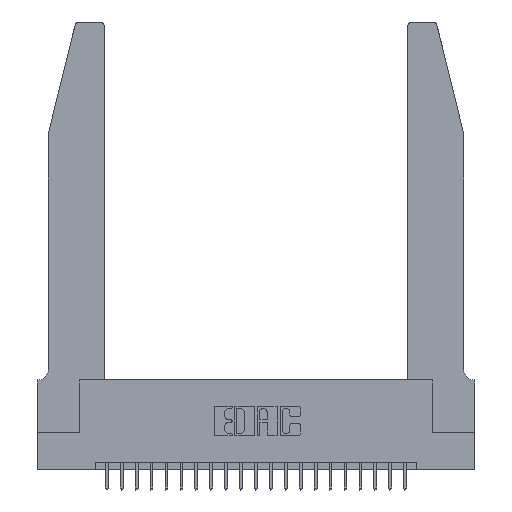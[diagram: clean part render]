
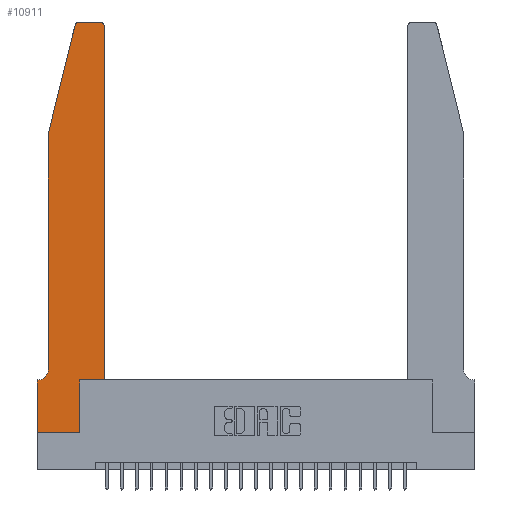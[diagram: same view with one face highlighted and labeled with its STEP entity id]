
A CAD part, top view. The second image highlights one B-rep face of the part: STEP entity #10911.
In plain terms, the highlighted planar face has unit normal (0, 0, 1).
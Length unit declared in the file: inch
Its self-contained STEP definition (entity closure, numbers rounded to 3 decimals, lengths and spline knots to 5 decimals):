
#308 = VERTEX_POINT ( 'NONE', #14367 ) ;
#468 = CARTESIAN_POINT ( 'NONE',  ( 0.2865, 0., 0.37 ) ) ;
#520 = VERTEX_POINT ( 'NONE', #7309 ) ;
#607 = FACE_OUTER_BOUND ( 'NONE', #18748, .T. ) ;
#777 = CARTESIAN_POINT ( 'NONE',  ( 0.0755, 2., 0.37 ) ) ;
#827 = ORIENTED_EDGE ( 'NONE', *, *, #13440, .T. ) ;
#828 = ORIENTED_EDGE ( 'NONE', *, *, #21350, .T. ) ;
#1389 = CARTESIAN_POINT ( 'NONE',  ( 0., 0.35, 0.37 ) ) ;
#1522 = ORIENTED_EDGE ( 'NONE', *, *, #9879, .T. ) ;
#1640 = LINE ( 'NONE', #20611, #9309 ) ;
#1994 = CIRCLE ( 'NONE', #5898, 0.03 ) ;
#2010 = CARTESIAN_POINT ( 'NONE',  ( 0.2605, 2.75, 0.37 ) ) ;
#2031 = CARTESIAN_POINT ( 'NONE',  ( 0., 0., 0.37 ) ) ;
#2139 = ORIENTED_EDGE ( 'NONE', *, *, #13582, .T. ) ;
#2393 = DIRECTION ( 'NONE',  ( 0., 0., -1. ) ) ;
#2446 = ORIENTED_EDGE ( 'NONE', *, *, #19877, .T. ) ;
#3504 = VECTOR ( 'NONE', #11298, 39.37008 ) ;
#3564 = EDGE_CURVE ( 'NONE', #520, #5819, #19365, .T. ) ;
#4402 = PLANE ( 'NONE',  #9981 ) ;
#4574 = VERTEX_POINT ( 'NONE', #468 ) ;
#5304 = ORIENTED_EDGE ( 'NONE', *, *, #3564, .T. ) ;
#5811 = ORIENTED_EDGE ( 'NONE', *, *, #16252, .T. ) ;
#5819 = VERTEX_POINT ( 'NONE', #8015 ) ;
#5851 = CIRCLE ( 'NONE', #16009, 0.03 ) ;
#5898 = AXIS2_PLACEMENT_3D ( 'NONE', #21106, #11808, #18772 ) ;
#6084 = VECTOR ( 'NONE', #6490, 39.37008 ) ;
#6261 = CARTESIAN_POINT ( 'NONE',  ( 0.4505, 0.35, 0.37 ) ) ;
#6490 = DIRECTION ( 'NONE',  ( 0., -1., 0. ) ) ;
#7309 = CARTESIAN_POINT ( 'NONE',  ( 0.0755, 0.42, 0.37 ) ) ;
#7367 = DIRECTION ( 'NONE',  ( -0.239, -0.971, 0. ) ) ;
#7811 = EDGE_CURVE ( 'NONE', #308, #12737, #1640, .T. ) ;
#7961 = CARTESIAN_POINT ( 'NONE',  ( 0., 0.35, 0.37 ) ) ;
#8015 = CARTESIAN_POINT ( 'NONE',  ( 0.0055, 0.35, 0.37 ) ) ;
#8226 = DIRECTION ( 'NONE',  ( 0., 1., 0. ) ) ;
#8350 = VERTEX_POINT ( 'NONE', #10363 ) ;
#8658 = LINE ( 'NONE', #16139, #16761 ) ;
#8765 = DIRECTION ( 'NONE',  ( -1., 0., 0. ) ) ;
#8970 = ORIENTED_EDGE ( 'NONE', *, *, #22170, .T. ) ;
#9088 = VERTEX_POINT ( 'NONE', #13491 ) ;
#9309 = VECTOR ( 'NONE', #7367, 39.37008 ) ;
#9360 = ORIENTED_EDGE ( 'NONE', *, *, #16908, .T. ) ;
#9458 = DIRECTION ( 'NONE',  ( -1., 0., 0. ) ) ;
#9585 = LINE ( 'NONE', #6261, #21697 ) ;
#9609 = VECTOR ( 'NONE', #9458, 39.37008 ) ;
#9879 = EDGE_CURVE ( 'NONE', #8350, #10273, #9585, .T. ) ;
#9981 = AXIS2_PLACEMENT_3D ( 'NONE', #7961, #15685, #15196 ) ;
#10273 = VERTEX_POINT ( 'NONE', #16044 ) ;
#10363 = CARTESIAN_POINT ( 'NONE',  ( 0.4505, 0.35, 0.37 ) ) ;
#10710 = DIRECTION ( 'NONE',  ( 0., -1., 0. ) ) ;
#10911 = ADVANCED_FACE ( 'NONE', ( #607 ), #4402, .T. ) ;
#11044 = LINE ( 'NONE', #18856, #3504 ) ;
#11298 = DIRECTION ( 'NONE',  ( 0., 1., 0. ) ) ;
#11535 = CARTESIAN_POINT ( 'NONE',  ( 0.0755, 0.35, 0.37 ) ) ;
#11569 = AXIS2_PLACEMENT_3D ( 'NONE', #19142, #2393, #8765 ) ;
#11808 = DIRECTION ( 'NONE',  ( 0., 0., 1. ) ) ;
#12515 = VECTOR ( 'NONE', #17495, 39.37008 ) ;
#12737 = VERTEX_POINT ( 'NONE', #777 ) ;
#12916 = LINE ( 'NONE', #16358, #16746 ) ;
#13222 = LINE ( 'NONE', #17130, #20386 ) ;
#13440 = EDGE_CURVE ( 'NONE', #19111, #23696, #18757, .T. ) ;
#13491 = CARTESIAN_POINT ( 'NONE',  ( 0.2865, 0.35, 0.37 ) ) ;
#13582 = EDGE_CURVE ( 'NONE', #12737, #520, #23620, .T. ) ;
#14234 = ORIENTED_EDGE ( 'NONE', *, *, #17734, .T. ) ;
#14367 = CARTESIAN_POINT ( 'NONE',  ( 0.25487, 2.72718, 0.37 ) ) ;
#14754 = DIRECTION ( 'NONE',  ( 1., 0., 0. ) ) ;
#15132 = CARTESIAN_POINT ( 'NONE',  ( 0.4205, 2.75, 0.37 ) ) ;
#15196 = DIRECTION ( 'NONE',  ( 1., 0., 0. ) ) ;
#15685 = DIRECTION ( 'NONE',  ( 0., 0., 1. ) ) ;
#15788 = LINE ( 'NONE', #11535, #12515 ) ;
#16009 = AXIS2_PLACEMENT_3D ( 'NONE', #20029, #20148, #14754 ) ;
#16044 = CARTESIAN_POINT ( 'NONE',  ( 0.4505, 2.72, 0.37 ) ) ;
#16062 = ORIENTED_EDGE ( 'NONE', *, *, #7811, .T. ) ;
#16139 = CARTESIAN_POINT ( 'NONE',  ( 0., 0., 0.37 ) ) ;
#16184 = CARTESIAN_POINT ( 'NONE',  ( 0.0755, 2., 0.37 ) ) ;
#16252 = EDGE_CURVE ( 'NONE', #18072, #22385, #12916, .T. ) ;
#16358 = CARTESIAN_POINT ( 'NONE',  ( 0., 0., 0.37 ) ) ;
#16746 = VECTOR ( 'NONE', #10710, 39.37008 ) ;
#16761 = VECTOR ( 'NONE', #23573, 39.37008 ) ;
#16894 = DIRECTION ( 'NONE',  ( 1., 0., 0. ) ) ;
#16908 = EDGE_CURVE ( 'NONE', #22385, #4574, #8658, .T. ) ;
#17130 = CARTESIAN_POINT ( 'NONE',  ( 0.4505, 0.35, 0.37 ) ) ;
#17495 = DIRECTION ( 'NONE',  ( -1., 0., 0. ) ) ;
#17734 = EDGE_CURVE ( 'NONE', #10273, #19111, #5851, .T. ) ;
#17847 = CARTESIAN_POINT ( 'NONE',  ( 0.284, 2.75, 0.37 ) ) ;
#18072 = VERTEX_POINT ( 'NONE', #1389 ) ;
#18717 = EDGE_CURVE ( 'NONE', #5819, #18072, #15788, .T. ) ;
#18748 = EDGE_LOOP ( 'NONE', ( #827, #828, #16062, #2139, #5304, #22072, #5811, #9360, #2446, #8970, #1522, #14234 ) ) ;
#18757 = LINE ( 'NONE', #2010, #9609 ) ;
#18772 = DIRECTION ( 'NONE',  ( 1., 0., 0. ) ) ;
#18856 = CARTESIAN_POINT ( 'NONE',  ( 0.2865, 0.35, 0.37 ) ) ;
#19111 = VERTEX_POINT ( 'NONE', #15132 ) ;
#19142 = CARTESIAN_POINT ( 'NONE',  ( 0.0055, 0.42, 0.37 ) ) ;
#19365 = CIRCLE ( 'NONE', #11569, 0.07 ) ;
#19877 = EDGE_CURVE ( 'NONE', #4574, #9088, #11044, .T. ) ;
#20029 = CARTESIAN_POINT ( 'NONE',  ( 0.4205, 2.72, 0.37 ) ) ;
#20148 = DIRECTION ( 'NONE',  ( 0., 0., 1. ) ) ;
#20386 = VECTOR ( 'NONE', #16894, 39.37008 ) ;
#20611 = CARTESIAN_POINT ( 'NONE',  ( 0.0755, 2., 0.37 ) ) ;
#21106 = CARTESIAN_POINT ( 'NONE',  ( 0.284, 2.72, 0.37 ) ) ;
#21350 = EDGE_CURVE ( 'NONE', #23696, #308, #1994, .T. ) ;
#21697 = VECTOR ( 'NONE', #8226, 39.37008 ) ;
#22072 = ORIENTED_EDGE ( 'NONE', *, *, #18717, .T. ) ;
#22170 = EDGE_CURVE ( 'NONE', #9088, #8350, #13222, .T. ) ;
#22385 = VERTEX_POINT ( 'NONE', #2031 ) ;
#23573 = DIRECTION ( 'NONE',  ( 1., 0., 0. ) ) ;
#23620 = LINE ( 'NONE', #16184, #6084 ) ;
#23696 = VERTEX_POINT ( 'NONE', #17847 ) ;
